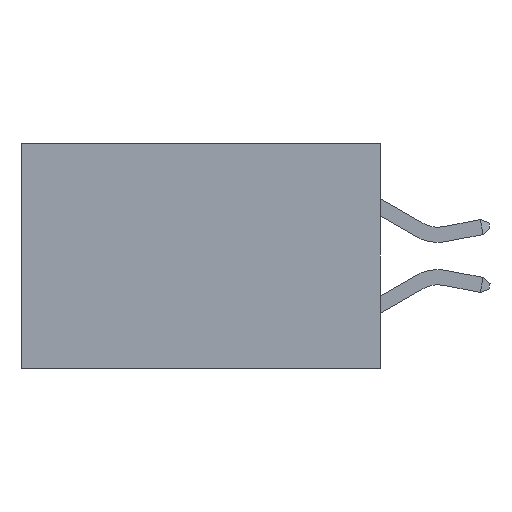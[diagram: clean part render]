
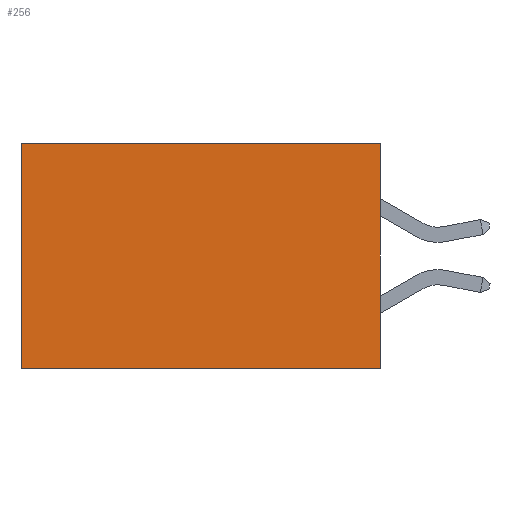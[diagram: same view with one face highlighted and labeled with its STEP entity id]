
A CAD part, left-side view. The second image highlights one B-rep face of the part: STEP entity #256.
In plain terms, the highlighted planar face has unit normal (-1, 0, 0).
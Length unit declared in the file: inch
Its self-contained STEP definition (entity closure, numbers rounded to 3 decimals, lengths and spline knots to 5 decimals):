
#18 = DIRECTION ( 'NONE',  ( 0., 1., 0. ) ) ;
#256 = ADVANCED_FACE ( 'NONE', ( #5685 ), #4531, .F. ) ;
#332 = VERTEX_POINT ( 'NONE', #4921 ) ;
#463 = EDGE_CURVE ( 'NONE', #7497, #1553, #6419, .T. ) ;
#808 = VECTOR ( 'NONE', #4467, 39.37008 ) ;
#946 = CARTESIAN_POINT ( 'NONE',  ( 0.277, 0.59, 0. ) ) ;
#1071 = CARTESIAN_POINT ( 'NONE',  ( 0.277, 0., 0. ) ) ;
#1553 = VERTEX_POINT ( 'NONE', #946 ) ;
#1622 = CARTESIAN_POINT ( 'NONE',  ( 0.277, 0., 0. ) ) ;
#1628 = VECTOR ( 'NONE', #18, 39.37008 ) ;
#1898 = LINE ( 'NONE', #6906, #7567 ) ;
#2024 = EDGE_LOOP ( 'NONE', ( #4296, #4304, #4365, #4381 ) ) ;
#2335 = VERTEX_POINT ( 'NONE', #6666 ) ;
#2564 = CARTESIAN_POINT ( 'NONE',  ( 0.277, 0.59, -0.37 ) ) ;
#4296 = ORIENTED_EDGE ( 'NONE', *, *, #8264, .T. ) ;
#4304 = ORIENTED_EDGE ( 'NONE', *, *, #7959, .F. ) ;
#4328 = EDGE_CURVE ( 'NONE', #7497, #332, #1898, .T. ) ;
#4365 = ORIENTED_EDGE ( 'NONE', *, *, #4328, .F. ) ;
#4381 = ORIENTED_EDGE ( 'NONE', *, *, #463, .T. ) ;
#4467 = DIRECTION ( 'NONE',  ( 0., 1., 0. ) ) ;
#4531 = PLANE ( 'NONE',  #8134 ) ;
#4627 = VECTOR ( 'NONE', #4704, 39.37008 ) ;
#4704 = DIRECTION ( 'NONE',  ( 0., 0., -1. ) ) ;
#4921 = CARTESIAN_POINT ( 'NONE',  ( 0.277, 0., -0.37 ) ) ;
#5685 = FACE_OUTER_BOUND ( 'NONE', #2024, .T. ) ;
#6285 = CARTESIAN_POINT ( 'NONE',  ( 0.277, 0., -0.37 ) ) ;
#6395 = LINE ( 'NONE', #2564, #4627 ) ;
#6419 = LINE ( 'NONE', #1622, #808 ) ;
#6666 = CARTESIAN_POINT ( 'NONE',  ( 0.277, 0.59, -0.37 ) ) ;
#6896 = DIRECTION ( 'NONE',  ( 0., 0., -1. ) ) ;
#6906 = CARTESIAN_POINT ( 'NONE',  ( 0.277, 0., -0.37 ) ) ;
#6923 = LINE ( 'NONE', #8327, #1628 ) ;
#7316 = DIRECTION ( 'NONE',  ( 1., 0., 0. ) ) ;
#7497 = VERTEX_POINT ( 'NONE', #1071 ) ;
#7567 = VECTOR ( 'NONE', #6896, 39.37008 ) ;
#7750 = DIRECTION ( 'NONE',  ( 0., 0., -1. ) ) ;
#7959 = EDGE_CURVE ( 'NONE', #332, #2335, #6923, .T. ) ;
#8134 = AXIS2_PLACEMENT_3D ( 'NONE', #6285, #7316, #7750 ) ;
#8264 = EDGE_CURVE ( 'NONE', #1553, #2335, #6395, .T. ) ;
#8327 = CARTESIAN_POINT ( 'NONE',  ( 0.277, 0., -0.37 ) ) ;
